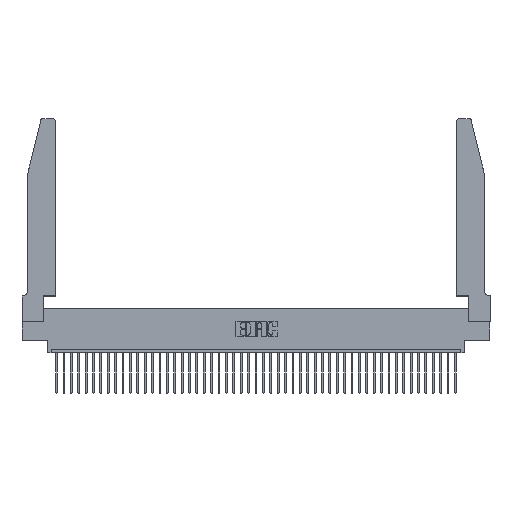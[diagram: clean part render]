
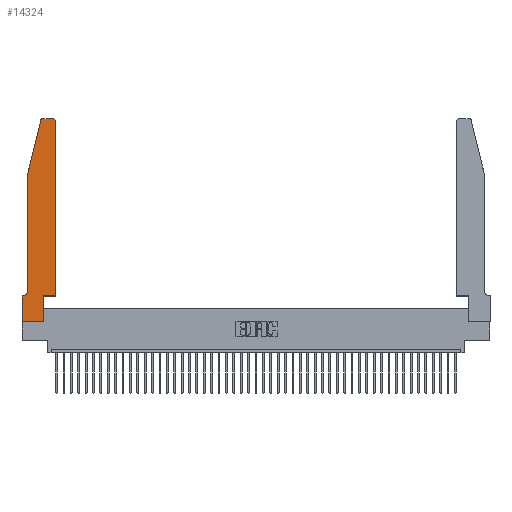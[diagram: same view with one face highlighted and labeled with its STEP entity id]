
A CAD part, top view. The second image highlights one B-rep face of the part: STEP entity #14324.
In plain terms, the highlighted planar face has unit normal (0, 0, 1).
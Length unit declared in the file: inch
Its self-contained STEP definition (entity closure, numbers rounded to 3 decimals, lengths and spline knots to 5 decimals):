
#172 = DIRECTION ( 'NONE',  ( 0., -1., 0. ) ) ;
#620 = ORIENTED_EDGE ( 'NONE', *, *, #41105, .T. ) ;
#1745 = EDGE_CURVE ( 'NONE', #6547, #3506, #26196, .T. ) ;
#1747 = DIRECTION ( 'NONE',  ( 1., 0., 0. ) ) ;
#2217 = CARTESIAN_POINT ( 'NONE',  ( 0.2865, 0.35, 0.37 ) ) ;
#2520 = ORIENTED_EDGE ( 'NONE', *, *, #21857, .T. ) ;
#3506 = VERTEX_POINT ( 'NONE', #43911 ) ;
#3713 = EDGE_CURVE ( 'NONE', #33989, #16572, #35625, .T. ) ;
#3905 = DIRECTION ( 'NONE',  ( 0., 0., 1. ) ) ;
#4723 = CARTESIAN_POINT ( 'NONE',  ( 0., 0., 0.37 ) ) ;
#5555 = VECTOR ( 'NONE', #11216, 39.37008 ) ;
#5760 = VECTOR ( 'NONE', #5768, 39.37008 ) ;
#5768 = DIRECTION ( 'NONE',  ( 1., 0., 0. ) ) ;
#5805 = CARTESIAN_POINT ( 'NONE',  ( 0.0055, 0.35, 0.37 ) ) ;
#5808 = DIRECTION ( 'NONE',  ( 0., 0., 1. ) ) ;
#5833 = ORIENTED_EDGE ( 'NONE', *, *, #3713, .T. ) ;
#6513 = CARTESIAN_POINT ( 'NONE',  ( 0.0055, 0.42, 0.37 ) ) ;
#6547 = VERTEX_POINT ( 'NONE', #40187 ) ;
#6695 = LINE ( 'NONE', #25025, #5555 ) ;
#7369 = LINE ( 'NONE', #22920, #5760 ) ;
#7639 = CARTESIAN_POINT ( 'NONE',  ( 0.4505, 0.35, 0.37 ) ) ;
#8642 = VERTEX_POINT ( 'NONE', #13687 ) ;
#9210 = ORIENTED_EDGE ( 'NONE', *, *, #1745, .T. ) ;
#9985 = EDGE_CURVE ( 'NONE', #18702, #22366, #31939, .T. ) ;
#10434 = AXIS2_PLACEMENT_3D ( 'NONE', #23106, #5808, #36606 ) ;
#11068 = DIRECTION ( 'NONE',  ( -0.239, -0.971, 0. ) ) ;
#11216 = DIRECTION ( 'NONE',  ( -1., 0., 0. ) ) ;
#11620 = LINE ( 'NONE', #2217, #31999 ) ;
#12104 = VECTOR ( 'NONE', #11068, 39.37008 ) ;
#13687 = CARTESIAN_POINT ( 'NONE',  ( 0.2865, 0., 0.37 ) ) ;
#13749 = CARTESIAN_POINT ( 'NONE',  ( 0.2865, 0.35, 0.37 ) ) ;
#14211 = EDGE_CURVE ( 'NONE', #19197, #18226, #29079, .T. ) ;
#14324 = ADVANCED_FACE ( 'NONE', ( #25289 ), #24559, .T. ) ;
#14389 = CARTESIAN_POINT ( 'NONE',  ( 0.0755, 0.35, 0.37 ) ) ;
#14632 = VECTOR ( 'NONE', #172, 39.37008 ) ;
#14665 = DIRECTION ( 'NONE',  ( -1., 0., 0. ) ) ;
#15903 = VERTEX_POINT ( 'NONE', #29008 ) ;
#16572 = VERTEX_POINT ( 'NONE', #40622 ) ;
#16819 = CARTESIAN_POINT ( 'NONE',  ( 0.4205, 2.75, 0.37 ) ) ;
#17273 = LINE ( 'NONE', #14389, #42492 ) ;
#18226 = VERTEX_POINT ( 'NONE', #40656 ) ;
#18345 = DIRECTION ( 'NONE',  ( 0., 0., 1. ) ) ;
#18394 = LINE ( 'NONE', #20820, #14632 ) ;
#18494 = DIRECTION ( 'NONE',  ( 1., 0., 0. ) ) ;
#18702 = VERTEX_POINT ( 'NONE', #44031 ) ;
#19117 = EDGE_LOOP ( 'NONE', ( #35381, #9210, #620, #23008, #28379, #29319, #5833, #35055, #2520, #44424, #24730, #19484 ) ) ;
#19197 = VERTEX_POINT ( 'NONE', #22346 ) ;
#19484 = ORIENTED_EDGE ( 'NONE', *, *, #21470, .T. ) ;
#20593 = VERTEX_POINT ( 'NONE', #13749 ) ;
#20820 = CARTESIAN_POINT ( 'NONE',  ( 0.0755, 2., 0.37 ) ) ;
#21470 = EDGE_CURVE ( 'NONE', #18226, #42584, #25669, .T. ) ;
#21857 = EDGE_CURVE ( 'NONE', #8642, #20593, #11620, .T. ) ;
#21980 = AXIS2_PLACEMENT_3D ( 'NONE', #29238, #3905, #26112 ) ;
#22346 = CARTESIAN_POINT ( 'NONE',  ( 0.4505, 0.35, 0.37 ) ) ;
#22366 = VERTEX_POINT ( 'NONE', #5805 ) ;
#22604 = LINE ( 'NONE', #7639, #25875 ) ;
#22920 = CARTESIAN_POINT ( 'NONE',  ( 0., 0., 0.37 ) ) ;
#23008 = ORIENTED_EDGE ( 'NONE', *, *, #41716, .T. ) ;
#23106 = CARTESIAN_POINT ( 'NONE',  ( 0.284, 2.72, 0.37 ) ) ;
#24559 = PLANE ( 'NONE',  #21980 ) ;
#24730 = ORIENTED_EDGE ( 'NONE', *, *, #14211, .T. ) ;
#25025 = CARTESIAN_POINT ( 'NONE',  ( 0.2605, 2.75, 0.37 ) ) ;
#25289 = FACE_OUTER_BOUND ( 'NONE', #19117, .T. ) ;
#25669 = CIRCLE ( 'NONE', #33701, 0.03 ) ;
#25875 = VECTOR ( 'NONE', #1747, 39.37008 ) ;
#26112 = DIRECTION ( 'NONE',  ( 1., 0., 0. ) ) ;
#26196 = CIRCLE ( 'NONE', #10434, 0.03 ) ;
#26606 = VECTOR ( 'NONE', #28983, 39.37008 ) ;
#26636 = EDGE_CURVE ( 'NONE', #20593, #19197, #22604, .T. ) ;
#27839 = DIRECTION ( 'NONE',  ( 0., 1., 0. ) ) ;
#28379 = ORIENTED_EDGE ( 'NONE', *, *, #9985, .T. ) ;
#28983 = DIRECTION ( 'NONE',  ( 0., -1., 0. ) ) ;
#29008 = CARTESIAN_POINT ( 'NONE',  ( 0.0755, 2., 0.37 ) ) ;
#29079 = LINE ( 'NONE', #41476, #33376 ) ;
#29238 = CARTESIAN_POINT ( 'NONE',  ( 0., 0.35, 0.37 ) ) ;
#29319 = ORIENTED_EDGE ( 'NONE', *, *, #34141, .T. ) ;
#29636 = AXIS2_PLACEMENT_3D ( 'NONE', #6513, #31499, #31641 ) ;
#30208 = DIRECTION ( 'NONE',  ( 0., 1., 0. ) ) ;
#30386 = LINE ( 'NONE', #31753, #12104 ) ;
#31499 = DIRECTION ( 'NONE',  ( 0., 0., -1. ) ) ;
#31641 = DIRECTION ( 'NONE',  ( -1., 0., 0. ) ) ;
#31753 = CARTESIAN_POINT ( 'NONE',  ( 0.0755, 2., 0.37 ) ) ;
#31939 = CIRCLE ( 'NONE', #29636, 0.07 ) ;
#31999 = VECTOR ( 'NONE', #30208, 39.37008 ) ;
#33376 = VECTOR ( 'NONE', #27839, 39.37008 ) ;
#33701 = AXIS2_PLACEMENT_3D ( 'NONE', #35183, #18345, #18494 ) ;
#33989 = VERTEX_POINT ( 'NONE', #37020 ) ;
#34141 = EDGE_CURVE ( 'NONE', #22366, #33989, #17273, .T. ) ;
#35055 = ORIENTED_EDGE ( 'NONE', *, *, #35945, .T. ) ;
#35183 = CARTESIAN_POINT ( 'NONE',  ( 0.4205, 2.72, 0.37 ) ) ;
#35381 = ORIENTED_EDGE ( 'NONE', *, *, #41116, .T. ) ;
#35625 = LINE ( 'NONE', #4723, #26606 ) ;
#35945 = EDGE_CURVE ( 'NONE', #16572, #8642, #7369, .T. ) ;
#36606 = DIRECTION ( 'NONE',  ( 1., 0., 0. ) ) ;
#37020 = CARTESIAN_POINT ( 'NONE',  ( 0., 0.35, 0.37 ) ) ;
#40187 = CARTESIAN_POINT ( 'NONE',  ( 0.284, 2.75, 0.37 ) ) ;
#40622 = CARTESIAN_POINT ( 'NONE',  ( 0., 0., 0.37 ) ) ;
#40656 = CARTESIAN_POINT ( 'NONE',  ( 0.4505, 2.72, 0.37 ) ) ;
#41105 = EDGE_CURVE ( 'NONE', #3506, #15903, #30386, .T. ) ;
#41116 = EDGE_CURVE ( 'NONE', #42584, #6547, #6695, .T. ) ;
#41476 = CARTESIAN_POINT ( 'NONE',  ( 0.4505, 0.35, 0.37 ) ) ;
#41716 = EDGE_CURVE ( 'NONE', #15903, #18702, #18394, .T. ) ;
#42492 = VECTOR ( 'NONE', #14665, 39.37008 ) ;
#42584 = VERTEX_POINT ( 'NONE', #16819 ) ;
#43911 = CARTESIAN_POINT ( 'NONE',  ( 0.25487, 2.72718, 0.37 ) ) ;
#44031 = CARTESIAN_POINT ( 'NONE',  ( 0.0755, 0.42, 0.37 ) ) ;
#44424 = ORIENTED_EDGE ( 'NONE', *, *, #26636, .T. ) ;
